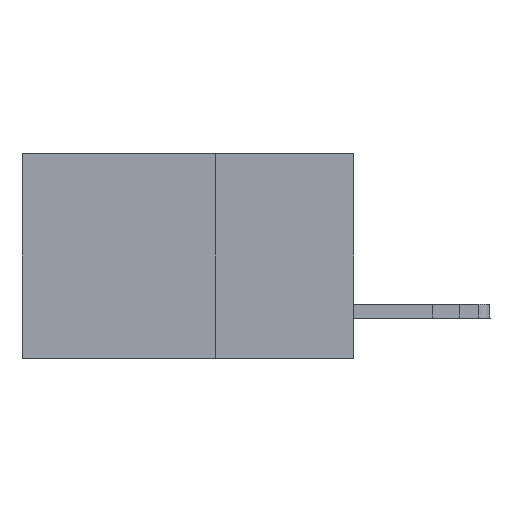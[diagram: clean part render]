
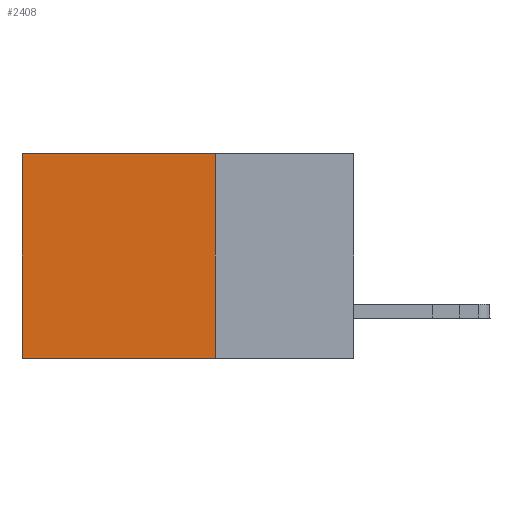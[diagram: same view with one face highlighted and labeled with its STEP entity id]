
A CAD part, left-side view. The second image highlights one B-rep face of the part: STEP entity #2408.
In plain terms, the highlighted planar face has unit normal (-1, 0, 0).
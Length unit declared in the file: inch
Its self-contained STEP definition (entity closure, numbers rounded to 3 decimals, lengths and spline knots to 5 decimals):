
#34 = VERTEX_POINT ( 'NONE', #22173 ) ;
#213 = PLANE ( 'NONE',  #22835 ) ;
#2037 = DIRECTION ( 'NONE',  ( 1., 0., 0. ) ) ;
#2258 = VECTOR ( 'NONE', #11157, 39.37008 ) ;
#2408 = ADVANCED_FACE ( 'NONE', ( #14975 ), #213, .F. ) ;
#2743 = CARTESIAN_POINT ( 'NONE',  ( 0.2875, 0.25, 0. ) ) ;
#4606 = VECTOR ( 'NONE', #15494, 39.37008 ) ;
#4632 = EDGE_CURVE ( 'NONE', #16757, #34, #19113, .T. ) ;
#5628 = VECTOR ( 'NONE', #17265, 39.37008 ) ;
#6150 = VERTEX_POINT ( 'NONE', #23247 ) ;
#7087 = LINE ( 'NONE', #21997, #2258 ) ;
#7165 = ORIENTED_EDGE ( 'NONE', *, *, #19402, .F. ) ;
#8167 = EDGE_CURVE ( 'NONE', #6150, #20375, #7087, .T. ) ;
#8397 = EDGE_CURVE ( 'NONE', #6150, #16757, #20130, .T. ) ;
#9659 = LINE ( 'NONE', #14245, #13922 ) ;
#11081 = CARTESIAN_POINT ( 'NONE',  ( 0.2875, 0.25, 0. ) ) ;
#11136 = ORIENTED_EDGE ( 'NONE', *, *, #8167, .F. ) ;
#11157 = DIRECTION ( 'NONE',  ( 0., 0., -1. ) ) ;
#11862 = CARTESIAN_POINT ( 'NONE',  ( 0.2875, 0.6, 0. ) ) ;
#13922 = VECTOR ( 'NONE', #19729, 39.37008 ) ;
#13982 = CARTESIAN_POINT ( 'NONE',  ( 0.2875, 0.25, -0.37 ) ) ;
#14245 = CARTESIAN_POINT ( 'NONE',  ( 0.2875, 0.25, -0.37 ) ) ;
#14741 = DIRECTION ( 'NONE',  ( 0., 0., -1. ) ) ;
#14975 = FACE_OUTER_BOUND ( 'NONE', #22869, .T. ) ;
#15494 = DIRECTION ( 'NONE',  ( 0., 0., -1. ) ) ;
#16757 = VERTEX_POINT ( 'NONE', #20833 ) ;
#17265 = DIRECTION ( 'NONE',  ( 0., 1., 0. ) ) ;
#19113 = LINE ( 'NONE', #11862, #4606 ) ;
#19402 = EDGE_CURVE ( 'NONE', #20375, #34, #9659, .T. ) ;
#19729 = DIRECTION ( 'NONE',  ( 0., 1., 0. ) ) ;
#20130 = LINE ( 'NONE', #2743, #5628 ) ;
#20375 = VERTEX_POINT ( 'NONE', #13982 ) ;
#20578 = ORIENTED_EDGE ( 'NONE', *, *, #4632, .T. ) ;
#20641 = ORIENTED_EDGE ( 'NONE', *, *, #8397, .T. ) ;
#20833 = CARTESIAN_POINT ( 'NONE',  ( 0.2875, 0.6, 0. ) ) ;
#21997 = CARTESIAN_POINT ( 'NONE',  ( 0.2875, 0.25, 0. ) ) ;
#22173 = CARTESIAN_POINT ( 'NONE',  ( 0.2875, 0.6, -0.37 ) ) ;
#22835 = AXIS2_PLACEMENT_3D ( 'NONE', #11081, #2037, #14741 ) ;
#22869 = EDGE_LOOP ( 'NONE', ( #20578, #7165, #11136, #20641 ) ) ;
#23247 = CARTESIAN_POINT ( 'NONE',  ( 0.2875, 0.25, 0. ) ) ;
